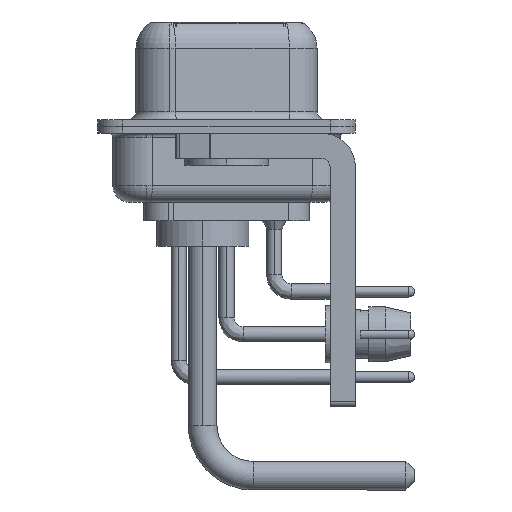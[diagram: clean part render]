
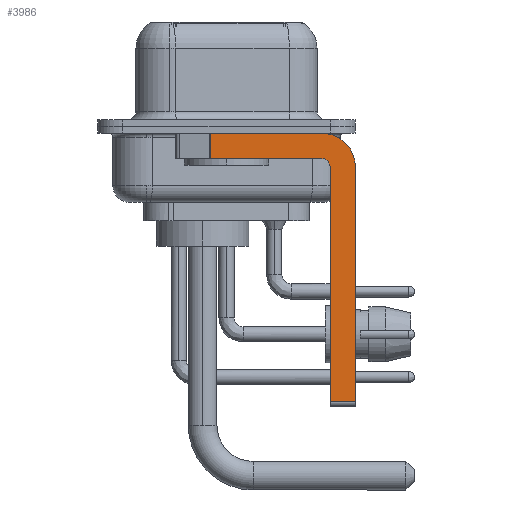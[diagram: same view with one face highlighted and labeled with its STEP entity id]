
A CAD part, left-side view. The second image highlights one B-rep face of the part: STEP entity #3986.
In plain terms, the highlighted planar face has unit normal (-1, 0, 0).
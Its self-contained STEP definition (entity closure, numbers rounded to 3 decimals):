
#1494 = VERTEX_POINT ( 'NONE', #27260 ) ;
#1557 = ORIENTED_EDGE ( 'NONE', *, *, #26505, .F. ) ;
#1677 = LINE ( 'NONE', #30747, #21687 ) ;
#1932 = FACE_OUTER_BOUND ( 'NONE', #27686, .T. ) ;
#2820 = LINE ( 'NONE', #19688, #17426 ) ;
#3986 = ADVANCED_FACE ( 'NONE', ( #1932 ), #26940, .F. ) ;
#4430 = ORIENTED_EDGE ( 'NONE', *, *, #29343, .T. ) ;
#4738 = LINE ( 'NONE', #9559, #17537 ) ;
#5673 = DIRECTION ( 'NONE',  ( 0., 0., -1. ) ) ;
#5991 = LINE ( 'NONE', #15810, #31718 ) ;
#6233 = LINE ( 'NONE', #30636, #26272 ) ;
#6238 = CARTESIAN_POINT ( 'NONE',  ( -2.9, -7.65, -16.35 ) ) ;
#6773 = VECTOR ( 'NONE', #22549, 1000. ) ;
#7202 = VERTEX_POINT ( 'NONE', #26729 ) ;
#7684 = CIRCLE ( 'NONE', #10227, 2. ) ;
#8311 = ORIENTED_EDGE ( 'NONE', *, *, #27829, .F. ) ;
#8581 = EDGE_CURVE ( 'NONE', #7202, #21904, #7684, .T. ) ;
#9535 = CARTESIAN_POINT ( 'NONE',  ( -2.9, -6.15, -16.35 ) ) ;
#9559 = CARTESIAN_POINT ( 'NONE',  ( -2.9, 3., -0.4 ) ) ;
#9728 = DIRECTION ( 'NONE',  ( 0., 0., 1. ) ) ;
#10184 = CARTESIAN_POINT ( 'NONE',  ( -2.9, -5.65, -1.9 ) ) ;
#10227 = AXIS2_PLACEMENT_3D ( 'NONE', #21340, #13641, #11392 ) ;
#10644 = EDGE_CURVE ( 'NONE', #23167, #7202, #4738, .T. ) ;
#11392 = DIRECTION ( 'NONE',  ( 0., 0., -1. ) ) ;
#11735 = DIRECTION ( 'NONE',  ( 0., 0., -1. ) ) ;
#13641 = DIRECTION ( 'NONE',  ( 1., 0., 0. ) ) ;
#14904 = CARTESIAN_POINT ( 'NONE',  ( -2.9, -5.65, -2.4 ) ) ;
#14997 = DIRECTION ( 'NONE',  ( 0., 0., 1. ) ) ;
#15518 = CARTESIAN_POINT ( 'NONE',  ( -2.9, -7.65, -2.4 ) ) ;
#15810 = CARTESIAN_POINT ( 'NONE',  ( -2.9, -7.65, -2.4 ) ) ;
#16226 = ORIENTED_EDGE ( 'NONE', *, *, #8581, .F. ) ;
#17179 = CARTESIAN_POINT ( 'NONE',  ( -2.9, -5.65, -1.9 ) ) ;
#17426 = VECTOR ( 'NONE', #9728, 1000. ) ;
#17437 = VERTEX_POINT ( 'NONE', #26198 ) ;
#17473 = ORIENTED_EDGE ( 'NONE', *, *, #29808, .F. ) ;
#17537 = VECTOR ( 'NONE', #24500, 1000. ) ;
#18597 = VERTEX_POINT ( 'NONE', #9535 ) ;
#19378 = CIRCLE ( 'NONE', #27597, 0.5 ) ;
#19554 = CARTESIAN_POINT ( 'NONE',  ( -2.9, 0.978, -0.4 ) ) ;
#19688 = CARTESIAN_POINT ( 'NONE',  ( -2.9, -6.15, -16.6 ) ) ;
#19930 = VERTEX_POINT ( 'NONE', #6238 ) ;
#21315 = ORIENTED_EDGE ( 'NONE', *, *, #30215, .T. ) ;
#21340 = CARTESIAN_POINT ( 'NONE',  ( -2.9, -5.65, -2.4 ) ) ;
#21687 = VECTOR ( 'NONE', #23363, 1000. ) ;
#21904 = VERTEX_POINT ( 'NONE', #15518 ) ;
#22442 = DIRECTION ( 'NONE',  ( 1., 0., 0. ) ) ;
#22549 = DIRECTION ( 'NONE',  ( 0., 1., 0. ) ) ;
#22748 = ORIENTED_EDGE ( 'NONE', *, *, #25724, .F. ) ;
#23167 = VERTEX_POINT ( 'NONE', #19554 ) ;
#23363 = DIRECTION ( 'NONE',  ( 0., -1., 0. ) ) ;
#24500 = DIRECTION ( 'NONE',  ( 0., -1., 0. ) ) ;
#24917 = DIRECTION ( 'NONE',  ( 0., 0., -1. ) ) ;
#24951 = DIRECTION ( 'NONE',  ( -1., 0., 0. ) ) ;
#25124 = LINE ( 'NONE', #10184, #6773 ) ;
#25558 = ORIENTED_EDGE ( 'NONE', *, *, #10644, .F. ) ;
#25724 = EDGE_CURVE ( 'NONE', #1494, #31323, #19378, .T. ) ;
#26198 = CARTESIAN_POINT ( 'NONE',  ( -2.9, 0.978, -1.9 ) ) ;
#26272 = VECTOR ( 'NONE', #24917, 1000. ) ;
#26505 = EDGE_CURVE ( 'NONE', #21904, #19930, #5991, .T. ) ;
#26729 = CARTESIAN_POINT ( 'NONE',  ( -2.9, -5.65, -0.4 ) ) ;
#26940 = PLANE ( 'NONE',  #30398 ) ;
#27260 = CARTESIAN_POINT ( 'NONE',  ( -2.9, -6.15, -2.4 ) ) ;
#27524 = CARTESIAN_POINT ( 'NONE',  ( -2.9, -5.65, -2.4 ) ) ;
#27597 = AXIS2_PLACEMENT_3D ( 'NONE', #27524, #24951, #14997 ) ;
#27686 = EDGE_LOOP ( 'NONE', ( #25558, #21315, #17473, #22748, #8311, #4430, #1557, #16226 ) ) ;
#27829 = EDGE_CURVE ( 'NONE', #18597, #1494, #2820, .T. ) ;
#29343 = EDGE_CURVE ( 'NONE', #18597, #19930, #1677, .T. ) ;
#29808 = EDGE_CURVE ( 'NONE', #31323, #17437, #25124, .T. ) ;
#30215 = EDGE_CURVE ( 'NONE', #23167, #17437, #6233, .T. ) ;
#30398 = AXIS2_PLACEMENT_3D ( 'NONE', #14904, #22442, #11735 ) ;
#30636 = CARTESIAN_POINT ( 'NONE',  ( -2.9, 0.978, -1.9 ) ) ;
#30747 = CARTESIAN_POINT ( 'NONE',  ( -2.9, -5.65, -16.35 ) ) ;
#31323 = VERTEX_POINT ( 'NONE', #17179 ) ;
#31718 = VECTOR ( 'NONE', #5673, 1000. ) ;
